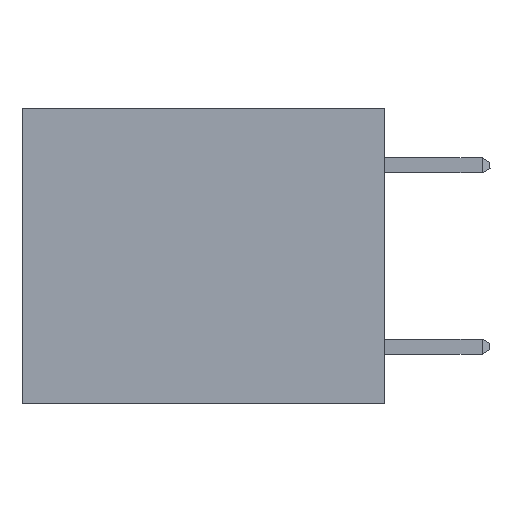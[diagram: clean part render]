
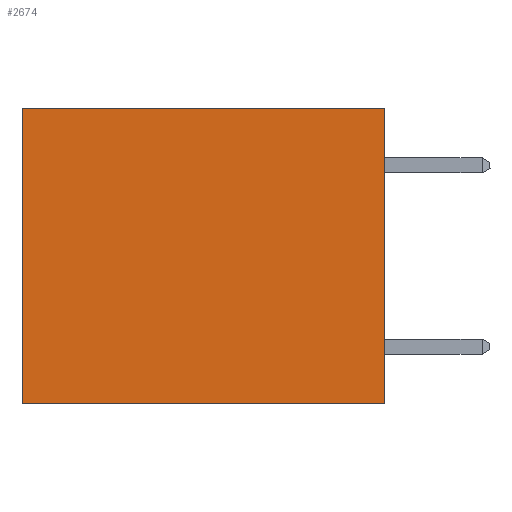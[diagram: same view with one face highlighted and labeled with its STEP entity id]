
A CAD part, left-side view. The second image highlights one B-rep face of the part: STEP entity #2674.
In plain terms, the highlighted planar face has unit normal (-1, 0, 0).
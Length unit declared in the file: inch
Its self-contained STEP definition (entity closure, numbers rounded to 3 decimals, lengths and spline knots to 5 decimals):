
#449 = ORIENTED_EDGE ( 'NONE', *, *, #19662, .T. ) ;
#1325 = VERTEX_POINT ( 'NONE', #20700 ) ;
#1454 = DIRECTION ( 'NONE',  ( 0., 0., -1. ) ) ;
#2016 = CARTESIAN_POINT ( 'NONE',  ( 0.3165, 0., 0. ) ) ;
#2522 = AXIS2_PLACEMENT_3D ( 'NONE', #15797, #23187, #25551 ) ;
#2674 = ADVANCED_FACE ( 'NONE', ( #25071 ), #6679, .F. ) ;
#3085 = CARTESIAN_POINT ( 'NONE',  ( 0.3165, 0., 0. ) ) ;
#5806 = EDGE_CURVE ( 'NONE', #14524, #11092, #26648, .T. ) ;
#6584 = VECTOR ( 'NONE', #1454, 39.37008 ) ;
#6679 = PLANE ( 'NONE',  #2522 ) ;
#8676 = DIRECTION ( 'NONE',  ( 0., 0., -1. ) ) ;
#9482 = CARTESIAN_POINT ( 'NONE',  ( 0.3165, 0., -0.49 ) ) ;
#10274 = VERTEX_POINT ( 'NONE', #26228 ) ;
#10470 = ORIENTED_EDGE ( 'NONE', *, *, #24763, .F. ) ;
#11092 = VERTEX_POINT ( 'NONE', #21566 ) ;
#11554 = VECTOR ( 'NONE', #8676, 39.37008 ) ;
#12816 = DIRECTION ( 'NONE',  ( 0., 1., 0. ) ) ;
#14524 = VERTEX_POINT ( 'NONE', #2016 ) ;
#15797 = CARTESIAN_POINT ( 'NONE',  ( 0.3165, 0., -0.49 ) ) ;
#17636 = VECTOR ( 'NONE', #21364, 39.37008 ) ;
#19224 = LINE ( 'NONE', #20261, #11554 ) ;
#19662 = EDGE_CURVE ( 'NONE', #11092, #10274, #24569, .T. ) ;
#19985 = CARTESIAN_POINT ( 'NONE',  ( 0.3165, 0.6, -0.49 ) ) ;
#20261 = CARTESIAN_POINT ( 'NONE',  ( 0.3165, 0., -0.49 ) ) ;
#20700 = CARTESIAN_POINT ( 'NONE',  ( 0.3165, 0., -0.49 ) ) ;
#21364 = DIRECTION ( 'NONE',  ( 0., 1., 0. ) ) ;
#21566 = CARTESIAN_POINT ( 'NONE',  ( 0.3165, 0.6, 0. ) ) ;
#21689 = LINE ( 'NONE', #9482, #17636 ) ;
#23187 = DIRECTION ( 'NONE',  ( 1., 0., 0. ) ) ;
#24569 = LINE ( 'NONE', #19985, #6584 ) ;
#24763 = EDGE_CURVE ( 'NONE', #1325, #10274, #21689, .T. ) ;
#24816 = VECTOR ( 'NONE', #12816, 39.37008 ) ;
#25071 = FACE_OUTER_BOUND ( 'NONE', #27731, .T. ) ;
#25197 = ORIENTED_EDGE ( 'NONE', *, *, #30158, .F. ) ;
#25551 = DIRECTION ( 'NONE',  ( 0., 0., -1. ) ) ;
#26071 = ORIENTED_EDGE ( 'NONE', *, *, #5806, .T. ) ;
#26228 = CARTESIAN_POINT ( 'NONE',  ( 0.3165, 0.6, -0.49 ) ) ;
#26648 = LINE ( 'NONE', #3085, #24816 ) ;
#27731 = EDGE_LOOP ( 'NONE', ( #449, #10470, #25197, #26071 ) ) ;
#30158 = EDGE_CURVE ( 'NONE', #14524, #1325, #19224, .T. ) ;
